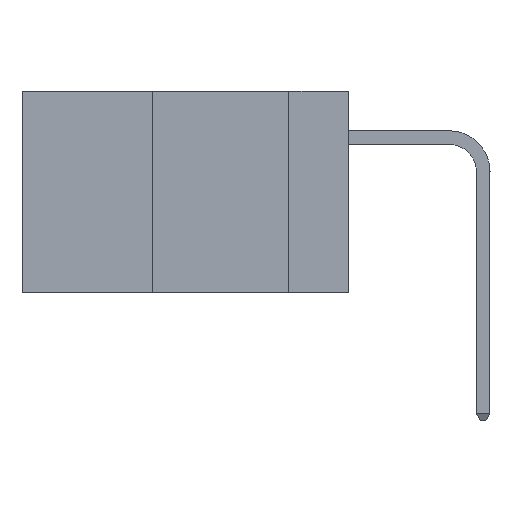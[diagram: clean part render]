
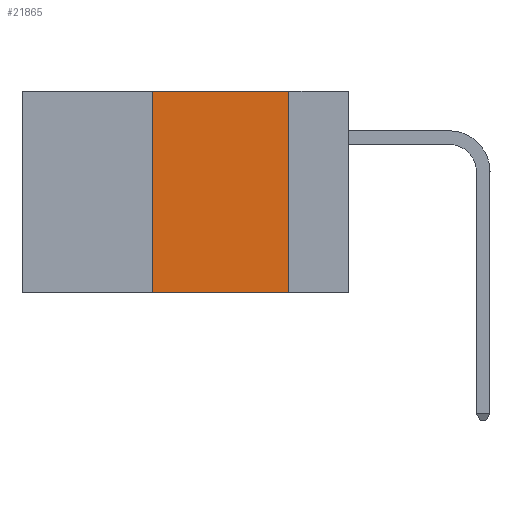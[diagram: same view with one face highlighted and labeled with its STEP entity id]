
A CAD part, left-side view. The second image highlights one B-rep face of the part: STEP entity #21865.
In plain terms, the highlighted planar face has unit normal (-1, 0, 0).
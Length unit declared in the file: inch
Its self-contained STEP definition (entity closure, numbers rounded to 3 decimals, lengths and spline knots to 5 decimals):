
#1168 = CARTESIAN_POINT ( 'NONE',  ( 0., 0.11, 0. ) ) ;
#1270 = CARTESIAN_POINT ( 'NONE',  ( 0., 0.36, -0.37 ) ) ;
#1631 = ORIENTED_EDGE ( 'NONE', *, *, #26959, .F. ) ;
#3304 = ORIENTED_EDGE ( 'NONE', *, *, #5221, .T. ) ;
#3552 = DIRECTION ( 'NONE',  ( 0., -1., 0. ) ) ;
#3771 = AXIS2_PLACEMENT_3D ( 'NONE', #25994, #28757, #12836 ) ;
#4861 = CARTESIAN_POINT ( 'NONE',  ( 0., 0.11, -0.37 ) ) ;
#4984 = ORIENTED_EDGE ( 'NONE', *, *, #30705, .F. ) ;
#5221 = EDGE_CURVE ( 'NONE', #19764, #25178, #14514, .T. ) ;
#6752 = EDGE_CURVE ( 'NONE', #19764, #28315, #21887, .T. ) ;
#6806 = CARTESIAN_POINT ( 'NONE',  ( 0., 0.36, 0. ) ) ;
#6940 = CARTESIAN_POINT ( 'NONE',  ( 0., 0.11, 0. ) ) ;
#8292 = LINE ( 'NONE', #19525, #28711 ) ;
#10170 = PLANE ( 'NONE',  #3771 ) ;
#10173 = VECTOR ( 'NONE', #25167, 39.37008 ) ;
#11007 = LINE ( 'NONE', #1168, #10173 ) ;
#11353 = CARTESIAN_POINT ( 'NONE',  ( 0., 0.36, 0. ) ) ;
#12836 = DIRECTION ( 'NONE',  ( 0., 0., -1. ) ) ;
#13283 = CARTESIAN_POINT ( 'NONE',  ( 0., 0.6, -0.37 ) ) ;
#13411 = DIRECTION ( 'NONE',  ( 0., -1., 0. ) ) ;
#14514 = LINE ( 'NONE', #13283, #33898 ) ;
#17197 = FACE_OUTER_BOUND ( 'NONE', #30456, .T. ) ;
#18642 = VERTEX_POINT ( 'NONE', #6940 ) ;
#19525 = CARTESIAN_POINT ( 'NONE',  ( 0., 0.6, 0. ) ) ;
#19764 = VERTEX_POINT ( 'NONE', #1270 ) ;
#21865 = ADVANCED_FACE ( 'NONE', ( #17197 ), #10170, .F. ) ;
#21887 = LINE ( 'NONE', #11353, #27282 ) ;
#22073 = DIRECTION ( 'NONE',  ( 0., 0., 1. ) ) ;
#23424 = ORIENTED_EDGE ( 'NONE', *, *, #6752, .F. ) ;
#25167 = DIRECTION ( 'NONE',  ( 0., 0., -1. ) ) ;
#25178 = VERTEX_POINT ( 'NONE', #4861 ) ;
#25994 = CARTESIAN_POINT ( 'NONE',  ( 0., 0.6, 0. ) ) ;
#26959 = EDGE_CURVE ( 'NONE', #18642, #25178, #11007, .T. ) ;
#27282 = VECTOR ( 'NONE', #22073, 39.37008 ) ;
#28315 = VERTEX_POINT ( 'NONE', #6806 ) ;
#28711 = VECTOR ( 'NONE', #3552, 39.37008 ) ;
#28757 = DIRECTION ( 'NONE',  ( 1., 0., 0. ) ) ;
#30456 = EDGE_LOOP ( 'NONE', ( #1631, #4984, #23424, #3304 ) ) ;
#30705 = EDGE_CURVE ( 'NONE', #28315, #18642, #8292, .T. ) ;
#33898 = VECTOR ( 'NONE', #13411, 39.37008 ) ;
